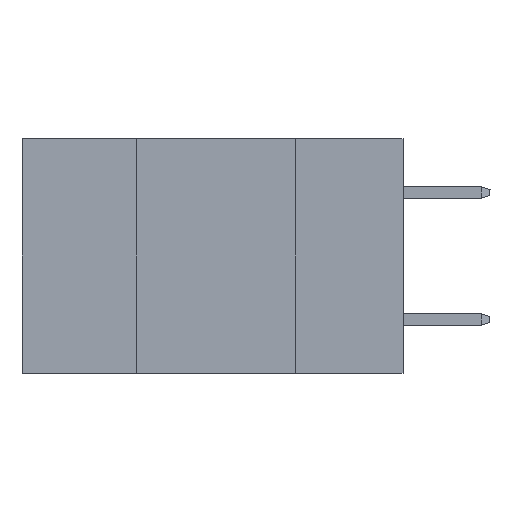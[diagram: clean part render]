
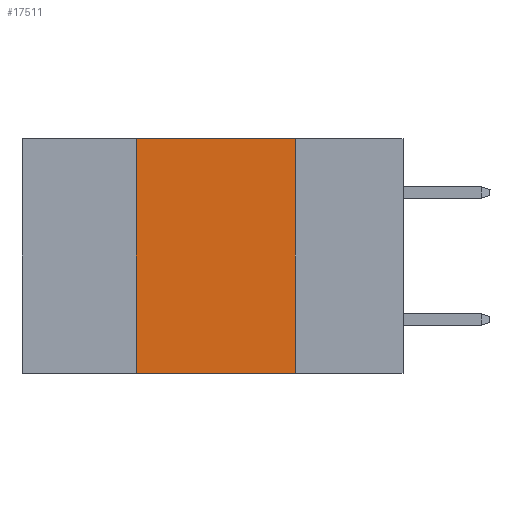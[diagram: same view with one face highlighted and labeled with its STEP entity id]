
A CAD part, left-side view. The second image highlights one B-rep face of the part: STEP entity #17511.
In plain terms, the highlighted planar face has unit normal (-1, 0, 0).
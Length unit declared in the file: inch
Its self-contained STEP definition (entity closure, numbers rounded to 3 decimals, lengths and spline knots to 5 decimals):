
#1249 = EDGE_CURVE ( 'NONE', #16167, #2763, #7238, .T. ) ;
#1406 = VECTOR ( 'NONE', #19061, 39.37008 ) ;
#2089 = CARTESIAN_POINT ( 'NONE',  ( 0., 0.17, -0.37 ) ) ;
#2459 = PLANE ( 'NONE',  #12311 ) ;
#2565 = VERTEX_POINT ( 'NONE', #2089 ) ;
#2763 = VERTEX_POINT ( 'NONE', #20467 ) ;
#3885 = EDGE_CURVE ( 'NONE', #9047, #16167, #7082, .T. ) ;
#5310 = EDGE_CURVE ( 'NONE', #2763, #2565, #16748, .T. ) ;
#7082 = LINE ( 'NONE', #14068, #18465 ) ;
#7111 = EDGE_LOOP ( 'NONE', ( #9620, #21241, #15534, #21151 ) ) ;
#7238 = LINE ( 'NONE', #13933, #1406 ) ;
#7316 = CARTESIAN_POINT ( 'NONE',  ( 0., 0.42, 0. ) ) ;
#8597 = DIRECTION ( 'NONE',  ( 0., 0., -1. ) ) ;
#9047 = VERTEX_POINT ( 'NONE', #10248 ) ;
#9620 = ORIENTED_EDGE ( 'NONE', *, *, #5310, .F. ) ;
#10248 = CARTESIAN_POINT ( 'NONE',  ( 0., 0.42, -0.37 ) ) ;
#10401 = CARTESIAN_POINT ( 'NONE',  ( 0., 0.6, 0. ) ) ;
#12230 = DIRECTION ( 'NONE',  ( 0., 0., -1. ) ) ;
#12311 = AXIS2_PLACEMENT_3D ( 'NONE', #10401, #18727, #12230 ) ;
#12406 = LINE ( 'NONE', #12624, #18950 ) ;
#12624 = CARTESIAN_POINT ( 'NONE',  ( 0., 0.6, -0.37 ) ) ;
#13474 = VECTOR ( 'NONE', #8597, 39.37008 ) ;
#13933 = CARTESIAN_POINT ( 'NONE',  ( 0., 0.6, 0. ) ) ;
#14068 = CARTESIAN_POINT ( 'NONE',  ( 0., 0.42, 0. ) ) ;
#14085 = DIRECTION ( 'NONE',  ( 0., -1., 0. ) ) ;
#15534 = ORIENTED_EDGE ( 'NONE', *, *, #3885, .F. ) ;
#16167 = VERTEX_POINT ( 'NONE', #7316 ) ;
#16434 = EDGE_CURVE ( 'NONE', #9047, #2565, #12406, .T. ) ;
#16748 = LINE ( 'NONE', #17167, #13474 ) ;
#17167 = CARTESIAN_POINT ( 'NONE',  ( 0., 0.17, 0. ) ) ;
#17511 = ADVANCED_FACE ( 'NONE', ( #19152 ), #2459, .F. ) ;
#18465 = VECTOR ( 'NONE', #20678, 39.37008 ) ;
#18727 = DIRECTION ( 'NONE',  ( 1., 0., 0. ) ) ;
#18950 = VECTOR ( 'NONE', #14085, 39.37008 ) ;
#19061 = DIRECTION ( 'NONE',  ( 0., -1., 0. ) ) ;
#19152 = FACE_OUTER_BOUND ( 'NONE', #7111, .T. ) ;
#20467 = CARTESIAN_POINT ( 'NONE',  ( 0., 0.17, 0. ) ) ;
#20678 = DIRECTION ( 'NONE',  ( 0., 0., 1. ) ) ;
#21151 = ORIENTED_EDGE ( 'NONE', *, *, #16434, .T. ) ;
#21241 = ORIENTED_EDGE ( 'NONE', *, *, #1249, .F. ) ;
